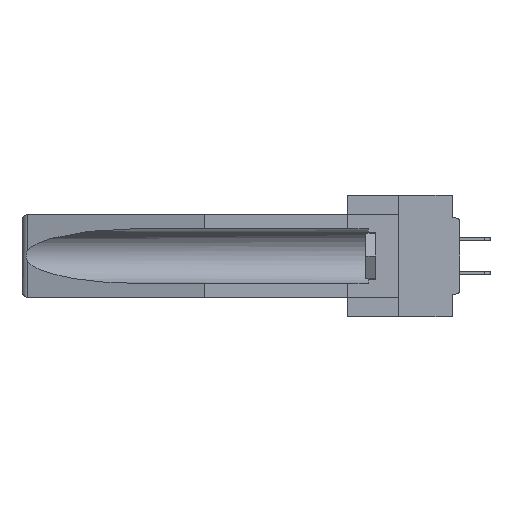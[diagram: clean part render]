
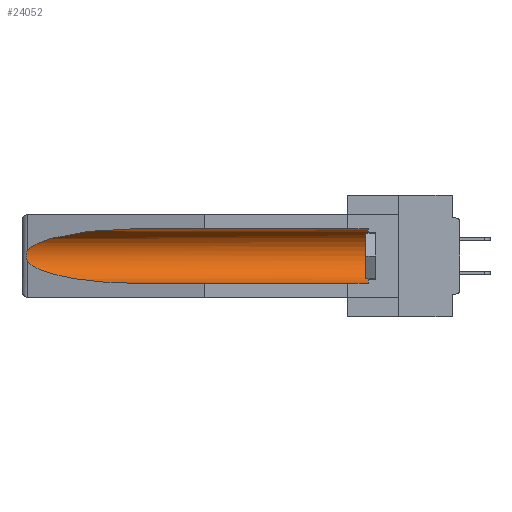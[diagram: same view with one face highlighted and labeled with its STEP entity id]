
A CAD part, left-side view. The second image highlights one B-rep face of the part: STEP entity #24052.
In plain terms, the highlighted cylindrical face has radius 2.857 mm (diameter 5.715 mm), a partial arc.
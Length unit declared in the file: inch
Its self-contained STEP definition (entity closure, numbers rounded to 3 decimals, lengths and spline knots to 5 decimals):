
#850 = CARTESIAN_POINT ( 'NONE',  ( 0.155, 1.07973, -0.059 ) ) ;
#1037 = CARTESIAN_POINT ( 'NONE',  ( 0.2673, 1.53269, -0.17917 ) ) ;
#2286 = LINE ( 'NONE', #6969, #7486 ) ;
#4072 = CARTESIAN_POINT ( 'NONE',  ( 0.155, 0.126, -0.1715 ) ) ;
#4511 = CARTESIAN_POINT ( 'NONE',  ( 0.26537, 1.52718, -0.19328 ) ) ;
#4673 = CARTESIAN_POINT ( 'NONE',  ( 0.2675, 1.53308, -0.16763 ) ) ;
#5111 = CARTESIAN_POINT ( 'NONE',  ( 0.26537, 1.52718, -0.19328 ) ) ;
#5820 = VERTEX_POINT ( 'NONE', #850 ) ;
#6502 = EDGE_CURVE ( 'NONE', #10085, #21316, #33216, .T. ) ;
#6969 = CARTESIAN_POINT ( 'NONE',  ( 0.155, -0.30754, -0.284 ) ) ;
#7324 = LINE ( 'NONE', #20413, #39484 ) ;
#7486 = VECTOR ( 'NONE', #33636, 39.37008 ) ;
#7512 = CARTESIAN_POINT ( 'NONE',  ( 0.155, 0.126, -0.059 ) ) ;
#7731 = CARTESIAN_POINT ( 'NONE',  ( 0.26597, 1.5296, -0.19026 ) ) ;
#7777 = CARTESIAN_POINT ( 'NONE',  ( 0.155, 1.07973, -0.059 ) ) ;
#8160 = CARTESIAN_POINT ( 'NONE',  ( 0.26537, 1.52718, -0.14972 ) ) ;
#8307 = CARTESIAN_POINT ( 'NONE',  ( 0.26654, 1.53092, -0.15636 ) ) ;
#8766 =( BOUNDED_CURVE ( )  B_SPLINE_CURVE ( 3, ( #7777, #11157, #11016, #37180 ),
 .UNSPECIFIED., .F., .F. ) 
 B_SPLINE_CURVE_WITH_KNOTS ( ( 4, 4 ),
 ( 4.71239, 6.08839 ),
 .UNSPECIFIED. ) 
 CURVE ( )  GEOMETRIC_REPRESENTATION_ITEM ( )  RATIONAL_B_SPLINE_CURVE ( ( 1., 0.848, 0.848, 1. ) ) 
 REPRESENTATION_ITEM ( '' )  );
#9405 = ORIENTED_EDGE ( 'NONE', *, *, #21615, .F. ) ;
#9707 = ORIENTED_EDGE ( 'NONE', *, *, #16364, .T. ) ;
#10085 = VERTEX_POINT ( 'NONE', #4511 ) ;
#10416 = VERTEX_POINT ( 'NONE', #7512 ) ;
#10726 = CARTESIAN_POINT ( 'NONE',  ( 0.25451, 1.48313, -0.24835 ) ) ;
#11016 = CARTESIAN_POINT ( 'NONE',  ( 0.25451, 1.48313, -0.09465 ) ) ;
#11039 = CARTESIAN_POINT ( 'NONE',  ( 0.155, 1.07973, -0.284 ) ) ;
#11157 = CARTESIAN_POINT ( 'NONE',  ( 0.21114, 1.30732, -0.059 ) ) ;
#11219 = B_SPLINE_CURVE_WITH_KNOTS ( 'NONE', 3,
 ( #8160, #34654, #8307, #14838, #4673, #40801, #1037, #24254, #7731, #5111 ),
 .UNSPECIFIED., .F., .F.,
 ( 4, 2, 2, 2, 4 ),
 ( 0., 0.00029, 0.00058, 0.00087, 0.00117 ),
 .UNSPECIFIED. ) ;
#11330 = CIRCLE ( 'NONE', #18186, 0.1125 ) ;
#13160 = FACE_OUTER_BOUND ( 'NONE', #23026, .T. ) ;
#13775 = CARTESIAN_POINT ( 'NONE',  ( 0.21114, 1.30732, -0.284 ) ) ;
#14838 = CARTESIAN_POINT ( 'NONE',  ( 0.2673, 1.5327, -0.16383 ) ) ;
#16364 = EDGE_CURVE ( 'NONE', #5820, #17224, #8766, .T. ) ;
#16598 = VERTEX_POINT ( 'NONE', #35507 ) ;
#17224 = VERTEX_POINT ( 'NONE', #20222 ) ;
#18186 = AXIS2_PLACEMENT_3D ( 'NONE', #4072, #30487, #40491 ) ;
#18443 = DIRECTION ( 'NONE',  ( 0., 1., 0. ) ) ;
#20222 = CARTESIAN_POINT ( 'NONE',  ( 0.26537, 1.52718, -0.14972 ) ) ;
#20413 = CARTESIAN_POINT ( 'NONE',  ( 0.155, -0.30754, -0.059 ) ) ;
#21316 = VERTEX_POINT ( 'NONE', #36687 ) ;
#21615 = EDGE_CURVE ( 'NONE', #16598, #21316, #2286, .T. ) ;
#21997 = EDGE_CURVE ( 'NONE', #17224, #10085, #11219, .T. ) ;
#22149 = AXIS2_PLACEMENT_3D ( 'NONE', #26995, #18443, #23124 ) ;
#23026 = EDGE_LOOP ( 'NONE', ( #9707, #38693, #36616, #9405, #26552, #41063 ) ) ;
#23124 = DIRECTION ( 'NONE',  ( 0., 0., 1. ) ) ;
#24052 = ADVANCED_FACE ( 'NONE', ( #13160 ), #36937, .F. ) ;
#24254 = CARTESIAN_POINT ( 'NONE',  ( 0.26655, 1.53094, -0.18657 ) ) ;
#25071 = EDGE_CURVE ( 'NONE', #10416, #5820, #7324, .T. ) ;
#26552 = ORIENTED_EDGE ( 'NONE', *, *, #39620, .T. ) ;
#26995 = CARTESIAN_POINT ( 'NONE',  ( 0.155, -0.30754, -0.1715 ) ) ;
#30487 = DIRECTION ( 'NONE',  ( 0., -1., 0. ) ) ;
#30872 = CARTESIAN_POINT ( 'NONE',  ( 0.26537, 1.52718, -0.19328 ) ) ;
#33216 =( BOUNDED_CURVE ( )  B_SPLINE_CURVE ( 3, ( #30872, #10726, #13775, #11039 ),
 .UNSPECIFIED., .F., .F. ) 
 B_SPLINE_CURVE_WITH_KNOTS ( ( 4, 4 ),
 ( 0.1948, 1.5708 ),
 .UNSPECIFIED. ) 
 CURVE ( )  GEOMETRIC_REPRESENTATION_ITEM ( )  RATIONAL_B_SPLINE_CURVE ( ( 1., 0.848, 0.848, 1. ) ) 
 REPRESENTATION_ITEM ( '' )  );
#33636 = DIRECTION ( 'NONE',  ( 0., 1., 0. ) ) ;
#34654 = CARTESIAN_POINT ( 'NONE',  ( 0.26597, 1.52961, -0.15275 ) ) ;
#35507 = CARTESIAN_POINT ( 'NONE',  ( 0.155, 0.126, -0.284 ) ) ;
#36616 = ORIENTED_EDGE ( 'NONE', *, *, #6502, .T. ) ;
#36687 = CARTESIAN_POINT ( 'NONE',  ( 0.155, 1.07973, -0.284 ) ) ;
#36937 = CYLINDRICAL_SURFACE ( 'NONE', #22149, 0.1125 ) ;
#37180 = CARTESIAN_POINT ( 'NONE',  ( 0.26537, 1.52718, -0.14972 ) ) ;
#38693 = ORIENTED_EDGE ( 'NONE', *, *, #21997, .T. ) ;
#39484 = VECTOR ( 'NONE', #39721, 39.37008 ) ;
#39620 = EDGE_CURVE ( 'NONE', #16598, #10416, #11330, .T. ) ;
#39721 = DIRECTION ( 'NONE',  ( 0., 1., 0. ) ) ;
#40491 = DIRECTION ( 'NONE',  ( 0., 0., 1. ) ) ;
#40801 = CARTESIAN_POINT ( 'NONE',  ( 0.2675, 1.53308, -0.17534 ) ) ;
#41063 = ORIENTED_EDGE ( 'NONE', *, *, #25071, .T. ) ;
